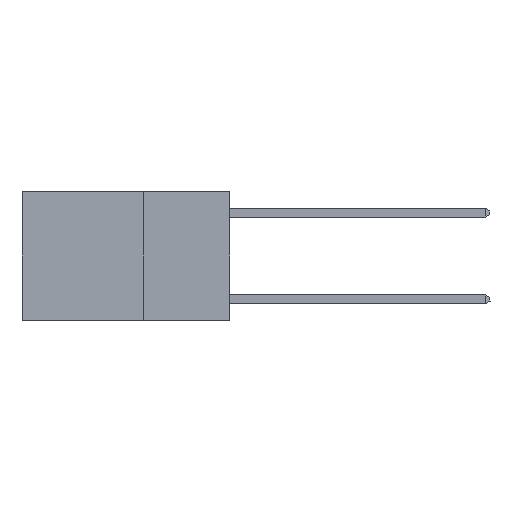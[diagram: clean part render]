
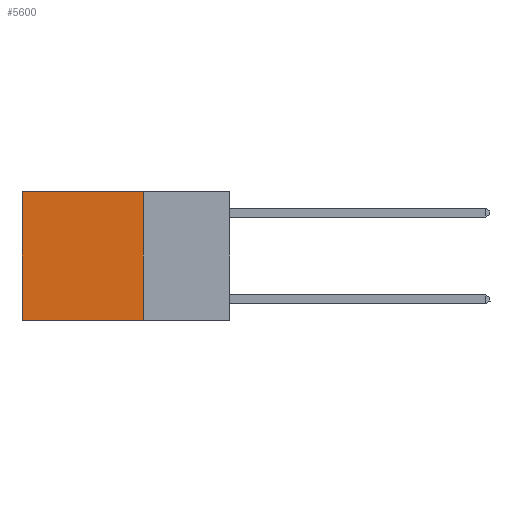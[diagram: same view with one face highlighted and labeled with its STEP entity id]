
A CAD part, left-side view. The second image highlights one B-rep face of the part: STEP entity #5600.
In plain terms, the highlighted planar face has unit normal (-1, 0, 0).
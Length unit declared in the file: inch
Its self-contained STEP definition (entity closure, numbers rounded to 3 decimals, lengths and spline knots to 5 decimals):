
#971 = CARTESIAN_POINT ( 'NONE',  ( 0.2625, 0.25, -0.37 ) ) ;
#1653 = DIRECTION ( 'NONE',  ( 0., 0., -1. ) ) ;
#2079 = VECTOR ( 'NONE', #1653, 39.37008 ) ;
#2832 = EDGE_LOOP ( 'NONE', ( #5919, #12199, #5631, #4053 ) ) ;
#2991 = CARTESIAN_POINT ( 'NONE',  ( 0.2625, 0.25, 0. ) ) ;
#3634 = VERTEX_POINT ( 'NONE', #13509 ) ;
#4053 = ORIENTED_EDGE ( 'NONE', *, *, #14998, .T. ) ;
#5600 = ADVANCED_FACE ( 'NONE', ( #5618 ), #16482, .F. ) ;
#5618 = FACE_OUTER_BOUND ( 'NONE', #2832, .T. ) ;
#5631 = ORIENTED_EDGE ( 'NONE', *, *, #16473, .F. ) ;
#5919 = ORIENTED_EDGE ( 'NONE', *, *, #6223, .T. ) ;
#5982 = CARTESIAN_POINT ( 'NONE',  ( 0.2625, 0.25, -0.37 ) ) ;
#6223 = EDGE_CURVE ( 'NONE', #6295, #18698, #11672, .T. ) ;
#6293 = VECTOR ( 'NONE', #15631, 39.37008 ) ;
#6295 = VERTEX_POINT ( 'NONE', #6894 ) ;
#6894 = CARTESIAN_POINT ( 'NONE',  ( 0.2625, 0.6, 0. ) ) ;
#7376 = EDGE_CURVE ( 'NONE', #15524, #18698, #13375, .T. ) ;
#8236 = DIRECTION ( 'NONE',  ( 0., 0., -1. ) ) ;
#8383 = DIRECTION ( 'NONE',  ( 1., 0., 0. ) ) ;
#9118 = VECTOR ( 'NONE', #14270, 39.37008 ) ;
#9939 = AXIS2_PLACEMENT_3D ( 'NONE', #13098, #8383, #8236 ) ;
#11672 = LINE ( 'NONE', #19344, #2079 ) ;
#12199 = ORIENTED_EDGE ( 'NONE', *, *, #7376, .F. ) ;
#13098 = CARTESIAN_POINT ( 'NONE',  ( 0.2625, 0.25, 0. ) ) ;
#13375 = LINE ( 'NONE', #971, #6293 ) ;
#13462 = LINE ( 'NONE', #2991, #9118 ) ;
#13509 = CARTESIAN_POINT ( 'NONE',  ( 0.2625, 0.25, 0. ) ) ;
#14270 = DIRECTION ( 'NONE',  ( 0., 1., 0. ) ) ;
#14642 = DIRECTION ( 'NONE',  ( 0., 0., -1. ) ) ;
#14789 = CARTESIAN_POINT ( 'NONE',  ( 0.2625, 0.25, 0. ) ) ;
#14998 = EDGE_CURVE ( 'NONE', #3634, #6295, #13462, .T. ) ;
#15524 = VERTEX_POINT ( 'NONE', #5982 ) ;
#15631 = DIRECTION ( 'NONE',  ( 0., 1., 0. ) ) ;
#16473 = EDGE_CURVE ( 'NONE', #3634, #15524, #16925, .T. ) ;
#16482 = PLANE ( 'NONE',  #9939 ) ;
#16925 = LINE ( 'NONE', #14789, #19683 ) ;
#17607 = CARTESIAN_POINT ( 'NONE',  ( 0.2625, 0.6, -0.37 ) ) ;
#18698 = VERTEX_POINT ( 'NONE', #17607 ) ;
#19344 = CARTESIAN_POINT ( 'NONE',  ( 0.2625, 0.6, 0. ) ) ;
#19683 = VECTOR ( 'NONE', #14642, 39.37008 ) ;
